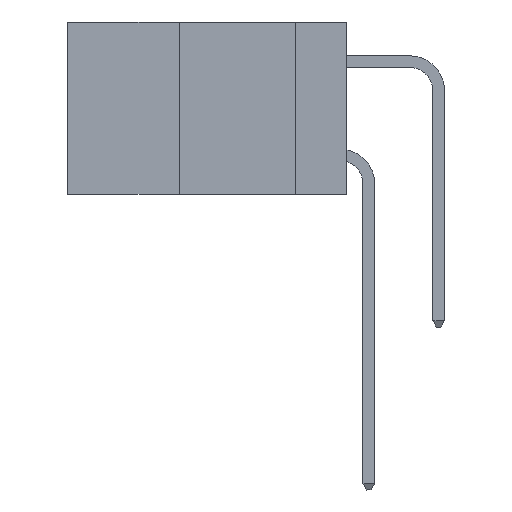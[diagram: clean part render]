
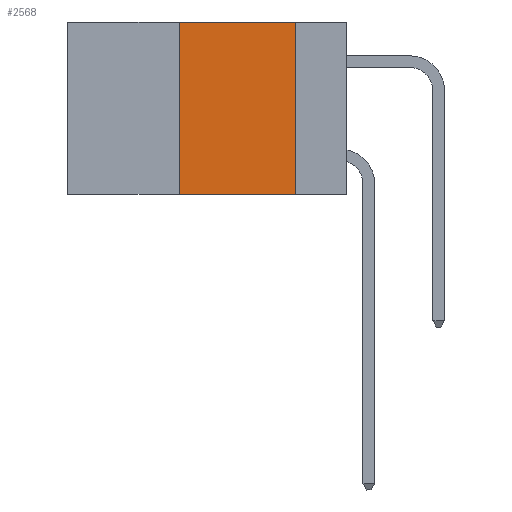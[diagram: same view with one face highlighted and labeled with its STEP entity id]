
A CAD part, left-side view. The second image highlights one B-rep face of the part: STEP entity #2568.
In plain terms, the highlighted planar face has unit normal (-1, 0, 0).
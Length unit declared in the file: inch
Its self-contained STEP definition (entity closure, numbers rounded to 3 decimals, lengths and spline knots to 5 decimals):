
#251 = EDGE_CURVE ( 'NONE', #8254, #5004, #3897, .T. ) ;
#927 = DIRECTION ( 'NONE',  ( 0., -1., 0. ) ) ;
#1810 = LINE ( 'NONE', #4985, #8178 ) ;
#2213 = DIRECTION ( 'NONE',  ( 0., 0., -1. ) ) ;
#2568 = ADVANCED_FACE ( 'NONE', ( #11031 ), #13979, .F. ) ;
#2604 = ORIENTED_EDGE ( 'NONE', *, *, #8596, .F. ) ;
#2618 = ORIENTED_EDGE ( 'NONE', *, *, #251, .F. ) ;
#2813 = CARTESIAN_POINT ( 'NONE',  ( 0., 0.11, 0. ) ) ;
#3682 = ORIENTED_EDGE ( 'NONE', *, *, #10830, .F. ) ;
#3897 = LINE ( 'NONE', #5585, #10527 ) ;
#4093 = ORIENTED_EDGE ( 'NONE', *, *, #12646, .T. ) ;
#4125 = CARTESIAN_POINT ( 'NONE',  ( 0., 0.36, -0.37 ) ) ;
#4985 = CARTESIAN_POINT ( 'NONE',  ( 0., 0.36, 0. ) ) ;
#5004 = VERTEX_POINT ( 'NONE', #15355 ) ;
#5585 = CARTESIAN_POINT ( 'NONE',  ( 0., 0.6, 0. ) ) ;
#6533 = VECTOR ( 'NONE', #14889, 39.37008 ) ;
#6579 = DIRECTION ( 'NONE',  ( 0., -1., 0. ) ) ;
#6626 = DIRECTION ( 'NONE',  ( 1., 0., 0. ) ) ;
#7257 = CARTESIAN_POINT ( 'NONE',  ( 0., 0.36, 0. ) ) ;
#7633 = VERTEX_POINT ( 'NONE', #11026 ) ;
#8178 = VECTOR ( 'NONE', #13283, 39.37008 ) ;
#8254 = VERTEX_POINT ( 'NONE', #7257 ) ;
#8596 = EDGE_CURVE ( 'NONE', #5004, #7633, #15894, .T. ) ;
#10527 = VECTOR ( 'NONE', #927, 39.37008 ) ;
#10830 = EDGE_CURVE ( 'NONE', #11034, #8254, #1810, .T. ) ;
#11026 = CARTESIAN_POINT ( 'NONE',  ( 0., 0.11, -0.37 ) ) ;
#11031 = FACE_OUTER_BOUND ( 'NONE', #14712, .T. ) ;
#11034 = VERTEX_POINT ( 'NONE', #4125 ) ;
#11486 = VECTOR ( 'NONE', #6579, 39.37008 ) ;
#12646 = EDGE_CURVE ( 'NONE', #11034, #7633, #14880, .T. ) ;
#13283 = DIRECTION ( 'NONE',  ( 0., 0., 1. ) ) ;
#13979 = PLANE ( 'NONE',  #14375 ) ;
#14030 = CARTESIAN_POINT ( 'NONE',  ( 0., 0.6, 0. ) ) ;
#14375 = AXIS2_PLACEMENT_3D ( 'NONE', #14030, #6626, #2213 ) ;
#14712 = EDGE_LOOP ( 'NONE', ( #2604, #2618, #3682, #4093 ) ) ;
#14824 = CARTESIAN_POINT ( 'NONE',  ( 0., 0.6, -0.37 ) ) ;
#14880 = LINE ( 'NONE', #14824, #11486 ) ;
#14889 = DIRECTION ( 'NONE',  ( 0., 0., -1. ) ) ;
#15355 = CARTESIAN_POINT ( 'NONE',  ( 0., 0.11, 0. ) ) ;
#15894 = LINE ( 'NONE', #2813, #6533 ) ;
